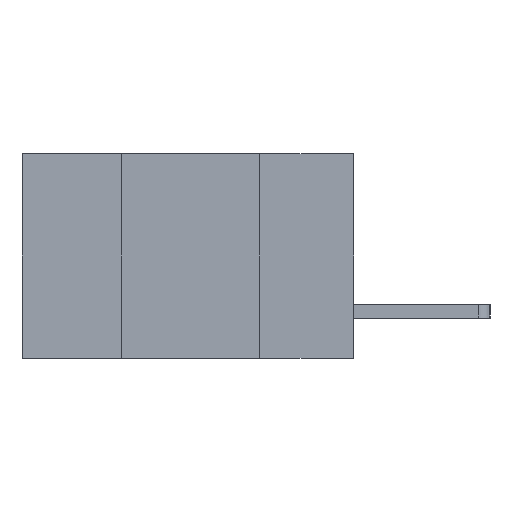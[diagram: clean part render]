
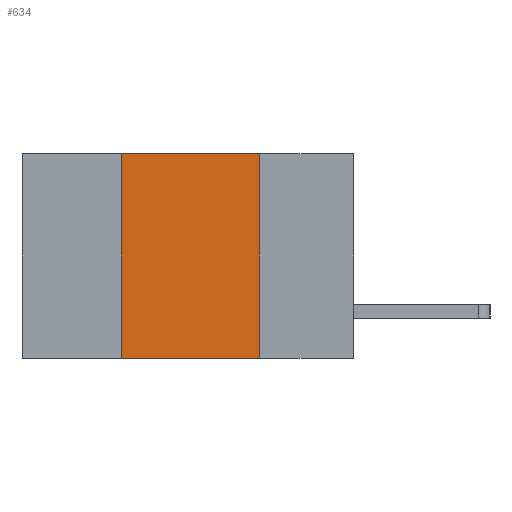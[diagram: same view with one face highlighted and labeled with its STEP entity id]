
A CAD part, left-side view. The second image highlights one B-rep face of the part: STEP entity #634.
In plain terms, the highlighted planar face has unit normal (-1, 0, 0).
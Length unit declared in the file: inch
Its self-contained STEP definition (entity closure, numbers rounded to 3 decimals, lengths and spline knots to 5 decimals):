
#231 = CARTESIAN_POINT ( 'NONE',  ( 0., 0.17, -0.37 ) ) ;
#634 = ADVANCED_FACE ( 'NONE', ( #9969 ), #1211, .F. ) ;
#1117 = LINE ( 'NONE', #7798, #2538 ) ;
#1211 = PLANE ( 'NONE',  #3998 ) ;
#1313 = CARTESIAN_POINT ( 'NONE',  ( 0., 0.42, 0. ) ) ;
#1533 = VERTEX_POINT ( 'NONE', #231 ) ;
#1976 = VERTEX_POINT ( 'NONE', #2293 ) ;
#2293 = CARTESIAN_POINT ( 'NONE',  ( 0., 0.17, 0. ) ) ;
#2378 = EDGE_CURVE ( 'NONE', #11393, #1533, #1117, .T. ) ;
#2380 = DIRECTION ( 'NONE',  ( 0., 0., -1. ) ) ;
#2538 = VECTOR ( 'NONE', #12094, 39.37008 ) ;
#3183 = CARTESIAN_POINT ( 'NONE',  ( 0., 0.6, 0. ) ) ;
#3998 = AXIS2_PLACEMENT_3D ( 'NONE', #3183, #4358, #6612 ) ;
#4015 = ORIENTED_EDGE ( 'NONE', *, *, #8207, .F. ) ;
#4045 = VECTOR ( 'NONE', #11539, 39.37008 ) ;
#4354 = CARTESIAN_POINT ( 'NONE',  ( 0., 0.17, 0. ) ) ;
#4358 = DIRECTION ( 'NONE',  ( 1., 0., 0. ) ) ;
#5014 = LINE ( 'NONE', #8378, #4045 ) ;
#5959 = VECTOR ( 'NONE', #13266, 39.37008 ) ;
#6219 = ORIENTED_EDGE ( 'NONE', *, *, #13710, .F. ) ;
#6442 = LINE ( 'NONE', #8633, #5959 ) ;
#6453 = EDGE_LOOP ( 'NONE', ( #4015, #6219, #13448, #9596 ) ) ;
#6612 = DIRECTION ( 'NONE',  ( 0., 0., -1. ) ) ;
#7798 = CARTESIAN_POINT ( 'NONE',  ( 0., 0.6, -0.37 ) ) ;
#8207 = EDGE_CURVE ( 'NONE', #1976, #1533, #12259, .T. ) ;
#8378 = CARTESIAN_POINT ( 'NONE',  ( 0., 0.42, 0. ) ) ;
#8633 = CARTESIAN_POINT ( 'NONE',  ( 0., 0.6, 0. ) ) ;
#9596 = ORIENTED_EDGE ( 'NONE', *, *, #2378, .T. ) ;
#9969 = FACE_OUTER_BOUND ( 'NONE', #6453, .T. ) ;
#10403 = EDGE_CURVE ( 'NONE', #11393, #13277, #5014, .T. ) ;
#11393 = VERTEX_POINT ( 'NONE', #12629 ) ;
#11539 = DIRECTION ( 'NONE',  ( 0., 0., 1. ) ) ;
#12024 = VECTOR ( 'NONE', #2380, 39.37008 ) ;
#12094 = DIRECTION ( 'NONE',  ( 0., -1., 0. ) ) ;
#12259 = LINE ( 'NONE', #4354, #12024 ) ;
#12629 = CARTESIAN_POINT ( 'NONE',  ( 0., 0.42, -0.37 ) ) ;
#13266 = DIRECTION ( 'NONE',  ( 0., -1., 0. ) ) ;
#13277 = VERTEX_POINT ( 'NONE', #1313 ) ;
#13448 = ORIENTED_EDGE ( 'NONE', *, *, #10403, .F. ) ;
#13710 = EDGE_CURVE ( 'NONE', #13277, #1976, #6442, .T. ) ;
